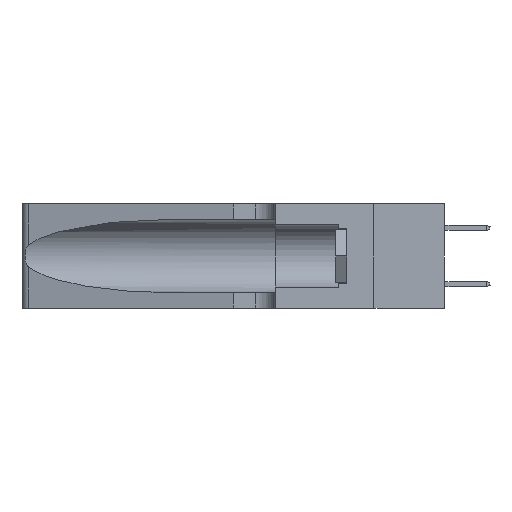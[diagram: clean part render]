
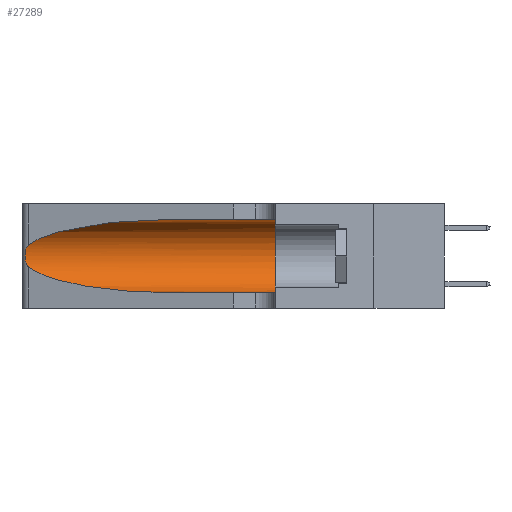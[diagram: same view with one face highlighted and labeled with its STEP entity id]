
A CAD part, left-side view. The second image highlights one B-rep face of the part: STEP entity #27289.
In plain terms, the highlighted cylindrical face has radius 3.308 mm (diameter 6.617 mm), a partial arc.
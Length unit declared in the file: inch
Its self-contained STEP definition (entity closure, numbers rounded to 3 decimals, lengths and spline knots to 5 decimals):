
#2880 = CARTESIAN_POINT ( 'NONE',  ( 0.26018, 1.23835, 0.19895 ) ) ;
#5046 = CARTESIAN_POINT ( 'NONE',  ( 0.2373, 1.15595, 0.28018 ) ) ;
#6602 = CARTESIAN_POINT ( 'NONE',  ( 0.26075, 1.23896, 0.178 ) ) ;
#6973 = EDGE_CURVE ( 'NONE', #46737, #43593, #42959, .T. ) ;
#7358 = VERTEX_POINT ( 'NONE', #19758 ) ;
#8353 = EDGE_CURVE ( 'NONE', #34460, #34825, #19287, .T. ) ;
#9632 = LINE ( 'NONE', #29797, #37848 ) ;
#10046 = CYLINDRICAL_SURFACE ( 'NONE', #18144, 0.13025 ) ;
#10346 = CARTESIAN_POINT ( 'NONE',  ( 0.25856, 1.23593, 0.16098 ) ) ;
#10885 = EDGE_CURVE ( 'NONE', #34825, #28202, #27915, .T. ) ;
#11009 = CARTESIAN_POINT ( 'NONE',  ( 0.1305, 0.35, 0.05475 ) ) ;
#13052 = CARTESIAN_POINT ( 'NONE',  ( 0.1305, 1.61858, 0.185 ) ) ;
#13885 = DIRECTION ( 'NONE',  ( 0., 1., 0. ) ) ;
#13935 = CARTESIAN_POINT ( 'NONE',  ( 0.25555, 1.22994, 0.2215 ) ) ;
#14093 = CARTESIAN_POINT ( 'NONE',  ( 0.25639, 1.23186, 0.15144 ) ) ;
#14413 = ORIENTED_EDGE ( 'NONE', *, *, #42742, .F. ) ;
#14948 =( BOUNDED_CURVE ( )  B_SPLINE_CURVE ( 3, ( #45294, #19908, #5046, #30951 ),
 .UNSPECIFIED., .F., .F. ) 
 B_SPLINE_CURVE_WITH_KNOTS ( ( 4, 4 ),
 ( 1.5708, 2.84003 ),
 .UNSPECIFIED. ) 
 CURVE ( )  GEOMETRIC_REPRESENTATION_ITEM ( )  RATIONAL_B_SPLINE_CURVE ( ( 1., 0.87, 0.87, 1. ) ) 
 REPRESENTATION_ITEM ( '' )  );
#15564 = ORIENTED_EDGE ( 'NONE', *, *, #6973, .F. ) ;
#15581 = LINE ( 'NONE', #43330, #44649 ) ;
#16836 = DIRECTION ( 'NONE',  ( 0., 0., -1. ) ) ;
#17891 = CARTESIAN_POINT ( 'NONE',  ( 0.25487, 1.22718, 0.14631 ) ) ;
#18144 = AXIS2_PLACEMENT_3D ( 'NONE', #13052, #42329, #16836 ) ;
#19262 = CARTESIAN_POINT ( 'NONE',  ( 0.25487, 1.22718, 0.22369 ) ) ;
#19287 = B_SPLINE_CURVE_WITH_KNOTS ( 'NONE', 3,
 ( #43189, #13935, #35944, #46822, #25163, #2880, #28820, #6602, #32449, #10346, #36105, #14093, #39710, #17891 ),
 .UNSPECIFIED., .F., .F.,
 ( 4, 2, 2, 2, 2, 2, 4 ),
 ( 0., 0.00027, 0.00053, 0.00107, 0.0016, 0.00187, 0.00214 ),
 .UNSPECIFIED. ) ;
#19758 = CARTESIAN_POINT ( 'NONE',  ( 0.1305, 0.72297, 0.31525 ) ) ;
#19908 = CARTESIAN_POINT ( 'NONE',  ( 0.18966, 0.96281, 0.31525 ) ) ;
#20925 = CARTESIAN_POINT ( 'NONE',  ( 0.18966, 0.96281, 0.05475 ) ) ;
#22903 = ORIENTED_EDGE ( 'NONE', *, *, #47103, .T. ) ;
#24300 = CARTESIAN_POINT ( 'NONE',  ( 0.25487, 1.22718, 0.14631 ) ) ;
#24891 = CARTESIAN_POINT ( 'NONE',  ( 0.25487, 1.22718, 0.14631 ) ) ;
#25163 = CARTESIAN_POINT ( 'NONE',  ( 0.25854, 1.2359, 0.20912 ) ) ;
#25316 = DIRECTION ( 'NONE',  ( 0., -1., 0. ) ) ;
#27289 = ADVANCED_FACE ( 'NONE', ( #29744 ), #10046, .F. ) ;
#27915 =( BOUNDED_CURVE ( )  B_SPLINE_CURVE ( 3, ( #24300, #46098, #20925, #46268 ),
 .UNSPECIFIED., .F., .F. ) 
 B_SPLINE_CURVE_WITH_KNOTS ( ( 4, 4 ),
 ( 3.44316, 4.71239 ),
 .UNSPECIFIED. ) 
 CURVE ( )  GEOMETRIC_REPRESENTATION_ITEM ( )  RATIONAL_B_SPLINE_CURVE ( ( 1., 0.87, 0.87, 1. ) ) 
 REPRESENTATION_ITEM ( '' )  );
#28161 = CARTESIAN_POINT ( 'NONE',  ( 0.1305, 0.72297, 0.05475 ) ) ;
#28202 = VERTEX_POINT ( 'NONE', #28161 ) ;
#28722 = AXIS2_PLACEMENT_3D ( 'NONE', #35894, #13885, #39525 ) ;
#28820 = CARTESIAN_POINT ( 'NONE',  ( 0.26075, 1.23896, 0.19203 ) ) ;
#28903 = CARTESIAN_POINT ( 'NONE',  ( 0.1305, 0.35, 0.31525 ) ) ;
#29744 = FACE_OUTER_BOUND ( 'NONE', #39254, .T. ) ;
#29797 = CARTESIAN_POINT ( 'NONE',  ( 0.1305, 1.61858, 0.31525 ) ) ;
#30951 = CARTESIAN_POINT ( 'NONE',  ( 0.25487, 1.22718, 0.22369 ) ) ;
#32449 = CARTESIAN_POINT ( 'NONE',  ( 0.26017, 1.23833, 0.17102 ) ) ;
#33428 = DIRECTION ( 'NONE',  ( 0., -1., 0. ) ) ;
#34460 = VERTEX_POINT ( 'NONE', #19262 ) ;
#34825 = VERTEX_POINT ( 'NONE', #24891 ) ;
#35894 = CARTESIAN_POINT ( 'NONE',  ( 0.1305, 0.35, 0.185 ) ) ;
#35944 = CARTESIAN_POINT ( 'NONE',  ( 0.25639, 1.23184, 0.21858 ) ) ;
#36105 = CARTESIAN_POINT ( 'NONE',  ( 0.25789, 1.23486, 0.15765 ) ) ;
#37085 = EDGE_CURVE ( 'NONE', #28202, #43593, #15581, .T. ) ;
#37848 = VECTOR ( 'NONE', #33428, 39.37008 ) ;
#39254 = EDGE_LOOP ( 'NONE', ( #22903, #46242, #39541, #44055, #15564, #14413 ) ) ;
#39525 = DIRECTION ( 'NONE',  ( 0., 0., 1. ) ) ;
#39541 = ORIENTED_EDGE ( 'NONE', *, *, #10885, .T. ) ;
#39710 = CARTESIAN_POINT ( 'NONE',  ( 0.25555, 1.22993, 0.14849 ) ) ;
#42329 = DIRECTION ( 'NONE',  ( 0., -1., 0. ) ) ;
#42742 = EDGE_CURVE ( 'NONE', #7358, #46737, #9632, .T. ) ;
#42959 = CIRCLE ( 'NONE', #28722, 0.13025 ) ;
#43189 = CARTESIAN_POINT ( 'NONE',  ( 0.25487, 1.22718, 0.22369 ) ) ;
#43330 = CARTESIAN_POINT ( 'NONE',  ( 0.1305, 1.61858, 0.05475 ) ) ;
#43593 = VERTEX_POINT ( 'NONE', #11009 ) ;
#44055 = ORIENTED_EDGE ( 'NONE', *, *, #37085, .T. ) ;
#44649 = VECTOR ( 'NONE', #25316, 39.37008 ) ;
#45294 = CARTESIAN_POINT ( 'NONE',  ( 0.1305, 0.72297, 0.31525 ) ) ;
#46098 = CARTESIAN_POINT ( 'NONE',  ( 0.2373, 1.15595, 0.08982 ) ) ;
#46242 = ORIENTED_EDGE ( 'NONE', *, *, #8353, .T. ) ;
#46268 = CARTESIAN_POINT ( 'NONE',  ( 0.1305, 0.72297, 0.05475 ) ) ;
#46737 = VERTEX_POINT ( 'NONE', #28903 ) ;
#46822 = CARTESIAN_POINT ( 'NONE',  ( 0.25787, 1.23484, 0.2124 ) ) ;
#47103 = EDGE_CURVE ( 'NONE', #7358, #34460, #14948, .T. ) ;
